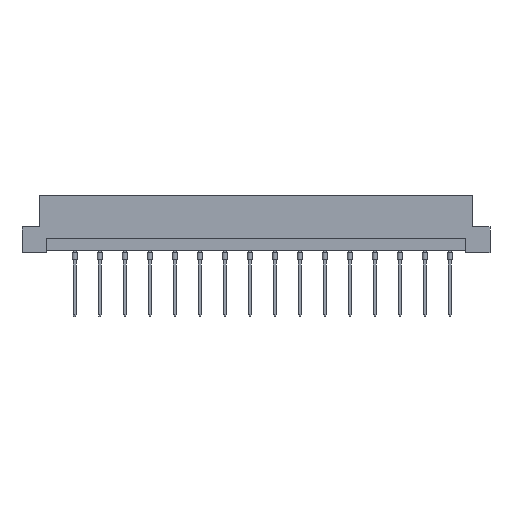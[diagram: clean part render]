
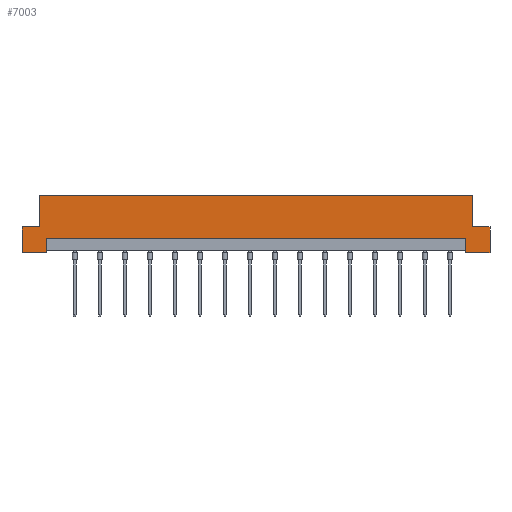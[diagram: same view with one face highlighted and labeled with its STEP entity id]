
A CAD part, front view. The second image highlights one B-rep face of the part: STEP entity #7003.
In plain terms, the highlighted planar face has unit normal (0, -1, 0).
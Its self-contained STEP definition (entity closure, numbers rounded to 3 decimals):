
#149 = LINE ( 'NONE', #8037, #15643 ) ;
#227 = VERTEX_POINT ( 'NONE', #15071 ) ;
#397 = VECTOR ( 'NONE', #15911, 1000. ) ;
#406 = CARTESIAN_POINT ( 'NONE',  ( -42.6, 0., 0.5 ) ) ;
#970 = ORIENTED_EDGE ( 'NONE', *, *, #9533, .F. ) ;
#1254 = EDGE_CURVE ( 'NONE', #7691, #15090, #11600, .T. ) ;
#1314 = LINE ( 'NONE', #15327, #6595 ) ;
#1712 = ORIENTED_EDGE ( 'NONE', *, *, #10133, .F. ) ;
#1782 = EDGE_CURVE ( 'NONE', #7691, #13736, #16486, .T. ) ;
#1895 = CARTESIAN_POINT ( 'NONE',  ( -47.5, 0., 0. ) ) ;
#1940 = VECTOR ( 'NONE', #10653, 1000. ) ;
#2520 = VECTOR ( 'NONE', #14714, 1000. ) ;
#2551 = CARTESIAN_POINT ( 'NONE',  ( -47.5, 0., 11.6 ) ) ;
#2610 = CARTESIAN_POINT ( 'NONE',  ( -47.5, 0., 0. ) ) ;
#2918 = VERTEX_POINT ( 'NONE', #6460 ) ;
#3148 = ORIENTED_EDGE ( 'NONE', *, *, #14098, .F. ) ;
#3262 = CARTESIAN_POINT ( 'NONE',  ( 42.6, 0., 0.5 ) ) ;
#3345 = EDGE_CURVE ( 'NONE', #227, #12201, #1314, .T. ) ;
#3634 = DIRECTION ( 'NONE',  ( -1., 0., 0. ) ) ;
#4210 = VECTOR ( 'NONE', #9173, 1000. ) ;
#4373 = ORIENTED_EDGE ( 'NONE', *, *, #11836, .F. ) ;
#4531 = DIRECTION ( 'NONE',  ( 0., 0., -1. ) ) ;
#4588 = ORIENTED_EDGE ( 'NONE', *, *, #11333, .F. ) ;
#4820 = EDGE_CURVE ( 'NONE', #10505, #5861, #7110, .T. ) ;
#5286 = EDGE_CURVE ( 'NONE', #13374, #10505, #6760, .T. ) ;
#5434 = CARTESIAN_POINT ( 'NONE',  ( -47.5, 0., 0. ) ) ;
#5438 = DIRECTION ( 'NONE',  ( 1., 0., 0. ) ) ;
#5498 = VERTEX_POINT ( 'NONE', #14798 ) ;
#5662 = VECTOR ( 'NONE', #14858, 1000. ) ;
#5827 = ORIENTED_EDGE ( 'NONE', *, *, #5286, .F. ) ;
#5861 = VERTEX_POINT ( 'NONE', #10154 ) ;
#5881 = EDGE_LOOP ( 'NONE', ( #970, #15849, #4588, #6560, #8080, #15382, #4373, #14726, #3148, #10600, #5827, #1712 ) ) ;
#6460 = CARTESIAN_POINT ( 'NONE',  ( 42.6, 0., 2.9 ) ) ;
#6499 = DIRECTION ( 'NONE',  ( 0., 0., 1. ) ) ;
#6560 = ORIENTED_EDGE ( 'NONE', *, *, #11485, .F. ) ;
#6562 = CARTESIAN_POINT ( 'NONE',  ( 44., 0., 5.2 ) ) ;
#6595 = VECTOR ( 'NONE', #15413, 1000. ) ;
#6760 = LINE ( 'NONE', #9525, #2520 ) ;
#6796 = LINE ( 'NONE', #406, #1940 ) ;
#6804 = VECTOR ( 'NONE', #7734, 1000. ) ;
#7003 = ADVANCED_FACE ( 'NONE', ( #14127 ), #15551, .F. ) ;
#7110 = LINE ( 'NONE', #1895, #397 ) ;
#7278 = VERTEX_POINT ( 'NONE', #7404 ) ;
#7404 = CARTESIAN_POINT ( 'NONE',  ( 47.5, 0., 0. ) ) ;
#7685 = CARTESIAN_POINT ( 'NONE',  ( 47.5, 0., 5.2 ) ) ;
#7691 = VERTEX_POINT ( 'NONE', #12248 ) ;
#7734 = DIRECTION ( 'NONE',  ( -1., 0., 0. ) ) ;
#8037 = CARTESIAN_POINT ( 'NONE',  ( -47.5, 0., 11.6 ) ) ;
#8080 = ORIENTED_EDGE ( 'NONE', *, *, #1782, .F. ) ;
#8138 = DIRECTION ( 'NONE',  ( 0., 0., -1. ) ) ;
#8144 = VECTOR ( 'NONE', #8138, 1000. ) ;
#9097 = LINE ( 'NONE', #15118, #14479 ) ;
#9173 = DIRECTION ( 'NONE',  ( 0., 0., 1. ) ) ;
#9225 = VECTOR ( 'NONE', #4531, 1000. ) ;
#9525 = CARTESIAN_POINT ( 'NONE',  ( -47.5, 0., 0. ) ) ;
#9533 = EDGE_CURVE ( 'NONE', #2918, #5498, #9097, .T. ) ;
#9834 = LINE ( 'NONE', #12337, #5662 ) ;
#10115 = DIRECTION ( 'NONE',  ( 0., 1., 0. ) ) ;
#10133 = EDGE_CURVE ( 'NONE', #5498, #13374, #6796, .T. ) ;
#10154 = CARTESIAN_POINT ( 'NONE',  ( -47.5, 0., 5.2 ) ) ;
#10505 = VERTEX_POINT ( 'NONE', #5434 ) ;
#10600 = ORIENTED_EDGE ( 'NONE', *, *, #4820, .F. ) ;
#10653 = DIRECTION ( 'NONE',  ( 0., 0., -1. ) ) ;
#11333 = EDGE_CURVE ( 'NONE', #7278, #13536, #14095, .T. ) ;
#11485 = EDGE_CURVE ( 'NONE', #13736, #7278, #15599, .T. ) ;
#11599 = EDGE_CURVE ( 'NONE', #2918, #13536, #14837, .T. ) ;
#11600 = LINE ( 'NONE', #6562, #4210 ) ;
#11775 = CARTESIAN_POINT ( 'NONE',  ( 44., 0., 11.6 ) ) ;
#11836 = EDGE_CURVE ( 'NONE', #12201, #15090, #149, .T. ) ;
#11996 = CARTESIAN_POINT ( 'NONE',  ( 47.5, 0., 0. ) ) ;
#12201 = VERTEX_POINT ( 'NONE', #12625 ) ;
#12248 = CARTESIAN_POINT ( 'NONE',  ( 44., 0., 5.2 ) ) ;
#12337 = CARTESIAN_POINT ( 'NONE',  ( -47.5, 0., 5.2 ) ) ;
#12525 = VECTOR ( 'NONE', #15056, 1000. ) ;
#12625 = CARTESIAN_POINT ( 'NONE',  ( -44., 0., 11.6 ) ) ;
#12875 = AXIS2_PLACEMENT_3D ( 'NONE', #2551, #10115, #6499 ) ;
#13374 = VERTEX_POINT ( 'NONE', #14052 ) ;
#13536 = VERTEX_POINT ( 'NONE', #14466 ) ;
#13736 = VERTEX_POINT ( 'NONE', #15122 ) ;
#14052 = CARTESIAN_POINT ( 'NONE',  ( -42.6, 0., 0. ) ) ;
#14095 = LINE ( 'NONE', #2610, #6804 ) ;
#14098 = EDGE_CURVE ( 'NONE', #5861, #227, #9834, .T. ) ;
#14127 = FACE_OUTER_BOUND ( 'NONE', #5881, .T. ) ;
#14466 = CARTESIAN_POINT ( 'NONE',  ( 42.6, 0., 0. ) ) ;
#14479 = VECTOR ( 'NONE', #3634, 1000. ) ;
#14714 = DIRECTION ( 'NONE',  ( -1., 0., 0. ) ) ;
#14726 = ORIENTED_EDGE ( 'NONE', *, *, #3345, .F. ) ;
#14798 = CARTESIAN_POINT ( 'NONE',  ( -42.6, 0., 2.9 ) ) ;
#14837 = LINE ( 'NONE', #3262, #9225 ) ;
#14858 = DIRECTION ( 'NONE',  ( 1., 0., 0. ) ) ;
#15056 = DIRECTION ( 'NONE',  ( 1., 0., 0. ) ) ;
#15071 = CARTESIAN_POINT ( 'NONE',  ( -44., 0., 5.2 ) ) ;
#15090 = VERTEX_POINT ( 'NONE', #11775 ) ;
#15118 = CARTESIAN_POINT ( 'NONE',  ( 42.6, 0., 2.9 ) ) ;
#15122 = CARTESIAN_POINT ( 'NONE',  ( 47.5, 0., 5.2 ) ) ;
#15327 = CARTESIAN_POINT ( 'NONE',  ( -44., 0., 5.2 ) ) ;
#15382 = ORIENTED_EDGE ( 'NONE', *, *, #1254, .T. ) ;
#15413 = DIRECTION ( 'NONE',  ( 0., 0., 1. ) ) ;
#15551 = PLANE ( 'NONE',  #12875 ) ;
#15599 = LINE ( 'NONE', #11996, #8144 ) ;
#15643 = VECTOR ( 'NONE', #5438, 1000. ) ;
#15849 = ORIENTED_EDGE ( 'NONE', *, *, #11599, .T. ) ;
#15911 = DIRECTION ( 'NONE',  ( 0., 0., 1. ) ) ;
#16486 = LINE ( 'NONE', #7685, #12525 ) ;
